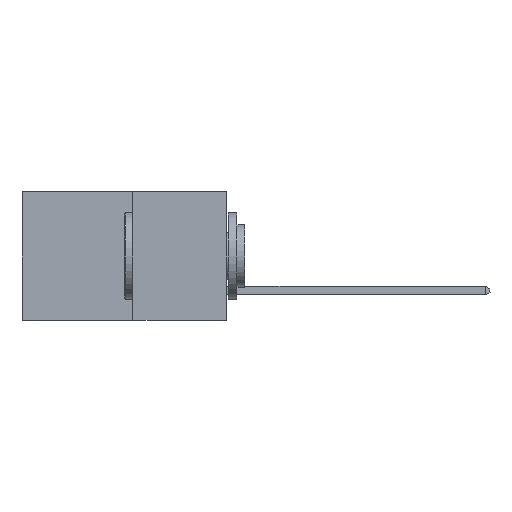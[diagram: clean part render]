
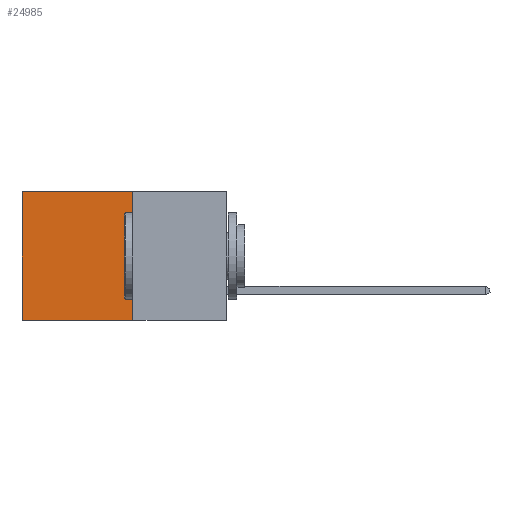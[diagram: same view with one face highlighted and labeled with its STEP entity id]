
A CAD part, left-side view. The second image highlights one B-rep face of the part: STEP entity #24985.
In plain terms, the highlighted planar face has unit normal (-1, 0, 0).
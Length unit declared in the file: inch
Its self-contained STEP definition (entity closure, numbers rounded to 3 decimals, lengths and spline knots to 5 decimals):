
#313 = LINE ( 'NONE', #12834, #12134 ) ;
#515 = VERTEX_POINT ( 'NONE', #25626 ) ;
#1034 = FACE_OUTER_BOUND ( 'NONE', #7507, .T. ) ;
#1564 = VECTOR ( 'NONE', #9993, 39.37008 ) ;
#1772 = DIRECTION ( 'NONE',  ( 0., 1., 0. ) ) ;
#2499 = DIRECTION ( 'NONE',  ( 0., 1., 0. ) ) ;
#2714 = PLANE ( 'NONE',  #13605 ) ;
#3145 = CARTESIAN_POINT ( 'NONE',  ( 0.277, 0.27, -0.37 ) ) ;
#4663 = ORIENTED_EDGE ( 'NONE', *, *, #24493, .F. ) ;
#4885 = ORIENTED_EDGE ( 'NONE', *, *, #7879, .T. ) ;
#4965 = DIRECTION ( 'NONE',  ( 1., 0., 0. ) ) ;
#6445 = CARTESIAN_POINT ( 'NONE',  ( 0.277, 0.59, 0. ) ) ;
#7507 = EDGE_LOOP ( 'NONE', ( #22840, #16168, #4663, #4885 ) ) ;
#7761 = CARTESIAN_POINT ( 'NONE',  ( 0.277, 0.59, -0.37 ) ) ;
#7879 = EDGE_CURVE ( 'NONE', #18014, #22140, #12339, .T. ) ;
#9341 = CARTESIAN_POINT ( 'NONE',  ( 0.277, 0.27, -0.37 ) ) ;
#9971 = DIRECTION ( 'NONE',  ( 0., 0., -1. ) ) ;
#9993 = DIRECTION ( 'NONE',  ( 0., 0., -1. ) ) ;
#12134 = VECTOR ( 'NONE', #1772, 39.37008 ) ;
#12339 = LINE ( 'NONE', #26608, #23287 ) ;
#12441 = VERTEX_POINT ( 'NONE', #21707 ) ;
#12825 = EDGE_CURVE ( 'NONE', #22140, #515, #19218, .T. ) ;
#12834 = CARTESIAN_POINT ( 'NONE',  ( 0.277, 0.27, -0.37 ) ) ;
#13532 = VECTOR ( 'NONE', #9971, 39.37008 ) ;
#13605 = AXIS2_PLACEMENT_3D ( 'NONE', #9341, #4965, #20393 ) ;
#16168 = ORIENTED_EDGE ( 'NONE', *, *, #18929, .F. ) ;
#18014 = VERTEX_POINT ( 'NONE', #18554 ) ;
#18554 = CARTESIAN_POINT ( 'NONE',  ( 0.277, 0.27, 0. ) ) ;
#18929 = EDGE_CURVE ( 'NONE', #12441, #515, #313, .T. ) ;
#19218 = LINE ( 'NONE', #7761, #1564 ) ;
#20393 = DIRECTION ( 'NONE',  ( 0., 0., -1. ) ) ;
#21707 = CARTESIAN_POINT ( 'NONE',  ( 0.277, 0.27, -0.37 ) ) ;
#22140 = VERTEX_POINT ( 'NONE', #6445 ) ;
#22840 = ORIENTED_EDGE ( 'NONE', *, *, #12825, .T. ) ;
#23287 = VECTOR ( 'NONE', #2499, 39.37008 ) ;
#24493 = EDGE_CURVE ( 'NONE', #18014, #12441, #25163, .T. ) ;
#24985 = ADVANCED_FACE ( 'NONE', ( #1034 ), #2714, .F. ) ;
#25163 = LINE ( 'NONE', #3145, #13532 ) ;
#25626 = CARTESIAN_POINT ( 'NONE',  ( 0.277, 0.59, -0.37 ) ) ;
#26608 = CARTESIAN_POINT ( 'NONE',  ( 0.277, 0.27, 0. ) ) ;
